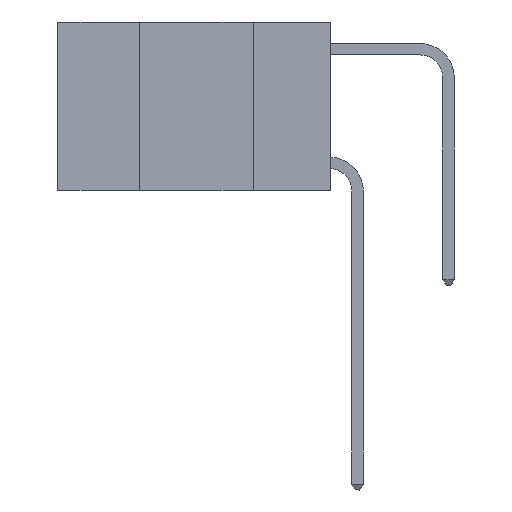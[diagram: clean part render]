
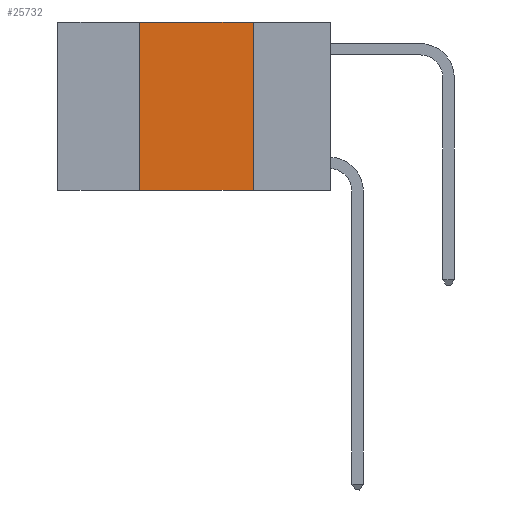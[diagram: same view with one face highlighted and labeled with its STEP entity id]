
A CAD part, left-side view. The second image highlights one B-rep face of the part: STEP entity #25732.
In plain terms, the highlighted planar face has unit normal (-1, 0, 0).
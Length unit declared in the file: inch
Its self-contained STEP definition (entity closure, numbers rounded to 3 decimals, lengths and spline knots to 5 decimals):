
#61 = LINE ( 'NONE', #8707, #7914 ) ;
#723 = EDGE_CURVE ( 'NONE', #8216, #3954, #24752, .T. ) ;
#2203 = EDGE_CURVE ( 'NONE', #21476, #3954, #61, .T. ) ;
#3378 = ORIENTED_EDGE ( 'NONE', *, *, #2203, .T. ) ;
#3542 = VECTOR ( 'NONE', #20275, 39.37008 ) ;
#3716 = PLANE ( 'NONE',  #23842 ) ;
#3954 = VERTEX_POINT ( 'NONE', #19050 ) ;
#3957 = ORIENTED_EDGE ( 'NONE', *, *, #5562, .F. ) ;
#4714 = VECTOR ( 'NONE', #24895, 39.37008 ) ;
#5562 = EDGE_CURVE ( 'NONE', #18356, #8216, #9987, .T. ) ;
#7062 = CARTESIAN_POINT ( 'NONE',  ( 0., 0.17, 0. ) ) ;
#7914 = VECTOR ( 'NONE', #19649, 39.37008 ) ;
#8216 = VERTEX_POINT ( 'NONE', #25707 ) ;
#8707 = CARTESIAN_POINT ( 'NONE',  ( 0., 0.6, -0.37 ) ) ;
#9463 = EDGE_CURVE ( 'NONE', #21476, #18356, #23193, .T. ) ;
#9987 = LINE ( 'NONE', #14235, #21812 ) ;
#12092 = DIRECTION ( 'NONE',  ( 0., 0., -1. ) ) ;
#13730 = CARTESIAN_POINT ( 'NONE',  ( 0., 0.42, -0.37 ) ) ;
#14235 = CARTESIAN_POINT ( 'NONE',  ( 0., 0.6, 0. ) ) ;
#16088 = CARTESIAN_POINT ( 'NONE',  ( 0., 0.6, 0. ) ) ;
#16218 = CARTESIAN_POINT ( 'NONE',  ( 0., 0.42, 0. ) ) ;
#16373 = FACE_OUTER_BOUND ( 'NONE', #26092, .T. ) ;
#18356 = VERTEX_POINT ( 'NONE', #16218 ) ;
#18646 = DIRECTION ( 'NONE',  ( 1., 0., 0. ) ) ;
#18986 = CARTESIAN_POINT ( 'NONE',  ( 0., 0.42, 0. ) ) ;
#19050 = CARTESIAN_POINT ( 'NONE',  ( 0., 0.17, -0.37 ) ) ;
#19649 = DIRECTION ( 'NONE',  ( 0., -1., 0. ) ) ;
#20104 = ORIENTED_EDGE ( 'NONE', *, *, #9463, .F. ) ;
#20275 = DIRECTION ( 'NONE',  ( 0., 0., -1. ) ) ;
#21476 = VERTEX_POINT ( 'NONE', #13730 ) ;
#21812 = VECTOR ( 'NONE', #22882, 39.37008 ) ;
#22882 = DIRECTION ( 'NONE',  ( 0., -1., 0. ) ) ;
#23193 = LINE ( 'NONE', #18986, #4714 ) ;
#23842 = AXIS2_PLACEMENT_3D ( 'NONE', #16088, #18646, #12092 ) ;
#24752 = LINE ( 'NONE', #7062, #3542 ) ;
#24895 = DIRECTION ( 'NONE',  ( 0., 0., 1. ) ) ;
#25707 = CARTESIAN_POINT ( 'NONE',  ( 0., 0.17, 0. ) ) ;
#25732 = ADVANCED_FACE ( 'NONE', ( #16373 ), #3716, .F. ) ;
#26092 = EDGE_LOOP ( 'NONE', ( #26360, #3957, #20104, #3378 ) ) ;
#26360 = ORIENTED_EDGE ( 'NONE', *, *, #723, .F. ) ;
